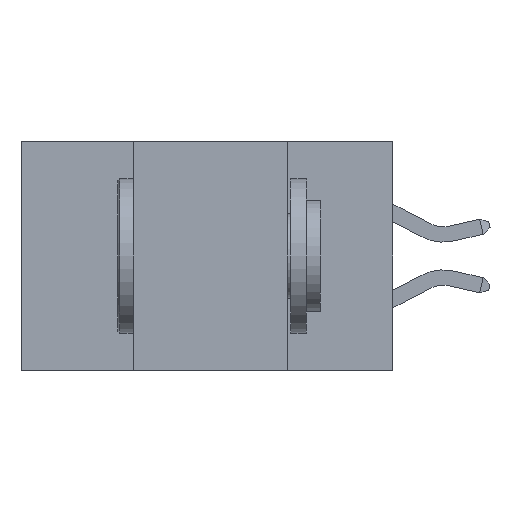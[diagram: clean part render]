
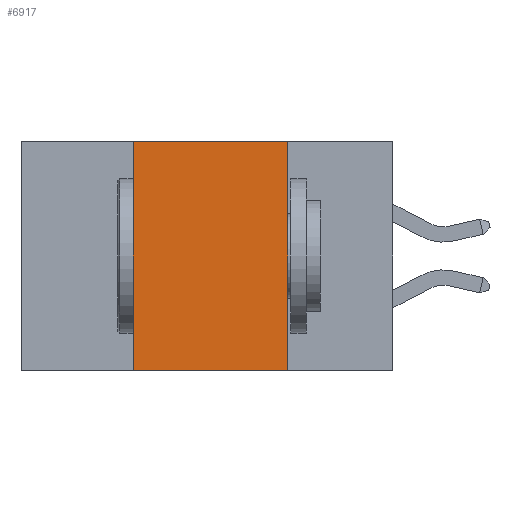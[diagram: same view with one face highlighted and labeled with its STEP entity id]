
A CAD part, left-side view. The second image highlights one B-rep face of the part: STEP entity #6917.
In plain terms, the highlighted planar face has unit normal (-1, 0, 0).
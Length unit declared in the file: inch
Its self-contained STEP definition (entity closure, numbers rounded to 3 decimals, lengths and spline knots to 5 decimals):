
#660 = VECTOR ( 'NONE', #10947, 39.37008 ) ;
#1397 = CARTESIAN_POINT ( 'NONE',  ( 0., 0.42, -0.37 ) ) ;
#1821 = VECTOR ( 'NONE', #13960, 39.37008 ) ;
#2863 = ORIENTED_EDGE ( 'NONE', *, *, #6909, .F. ) ;
#2945 = VERTEX_POINT ( 'NONE', #1397 ) ;
#3804 = FACE_OUTER_BOUND ( 'NONE', #12808, .T. ) ;
#4958 = CARTESIAN_POINT ( 'NONE',  ( 0., 0.42, 0. ) ) ;
#4995 = AXIS2_PLACEMENT_3D ( 'NONE', #10942, #10106, #10090 ) ;
#6909 = EDGE_CURVE ( 'NONE', #14402, #8915, #10139, .T. ) ;
#6917 = ADVANCED_FACE ( 'NONE', ( #3804 ), #10179, .F. ) ;
#7707 = VECTOR ( 'NONE', #7890, 39.37008 ) ;
#7890 = DIRECTION ( 'NONE',  ( 0., 0., 1. ) ) ;
#8915 = VERTEX_POINT ( 'NONE', #10567 ) ;
#8934 = ORIENTED_EDGE ( 'NONE', *, *, #9703, .F. ) ;
#9703 = EDGE_CURVE ( 'NONE', #2945, #14402, #10601, .T. ) ;
#9762 = CARTESIAN_POINT ( 'NONE',  ( 0., 0.17, 0. ) ) ;
#10090 = DIRECTION ( 'NONE',  ( 0., 0., -1. ) ) ;
#10106 = DIRECTION ( 'NONE',  ( 1., 0., 0. ) ) ;
#10139 = LINE ( 'NONE', #10422, #660 ) ;
#10179 = PLANE ( 'NONE',  #4995 ) ;
#10422 = CARTESIAN_POINT ( 'NONE',  ( 0., 0.6, 0. ) ) ;
#10567 = CARTESIAN_POINT ( 'NONE',  ( 0., 0.17, 0. ) ) ;
#10601 = LINE ( 'NONE', #12152, #7707 ) ;
#10791 = CARTESIAN_POINT ( 'NONE',  ( 0., 0.6, -0.37 ) ) ;
#10942 = CARTESIAN_POINT ( 'NONE',  ( 0., 0.6, 0. ) ) ;
#10947 = DIRECTION ( 'NONE',  ( 0., -1., 0. ) ) ;
#11433 = ORIENTED_EDGE ( 'NONE', *, *, #12025, .F. ) ;
#11765 = ORIENTED_EDGE ( 'NONE', *, *, #12648, .T. ) ;
#12025 = EDGE_CURVE ( 'NONE', #8915, #13913, #13830, .T. ) ;
#12152 = CARTESIAN_POINT ( 'NONE',  ( 0., 0.42, 0. ) ) ;
#12648 = EDGE_CURVE ( 'NONE', #2945, #13913, #13645, .T. ) ;
#12808 = EDGE_LOOP ( 'NONE', ( #11433, #2863, #8934, #11765 ) ) ;
#12944 = DIRECTION ( 'NONE',  ( 0., 0., -1. ) ) ;
#13494 = VECTOR ( 'NONE', #12944, 39.37008 ) ;
#13645 = LINE ( 'NONE', #10791, #1821 ) ;
#13701 = CARTESIAN_POINT ( 'NONE',  ( 0., 0.17, -0.37 ) ) ;
#13830 = LINE ( 'NONE', #9762, #13494 ) ;
#13913 = VERTEX_POINT ( 'NONE', #13701 ) ;
#13960 = DIRECTION ( 'NONE',  ( 0., -1., 0. ) ) ;
#14402 = VERTEX_POINT ( 'NONE', #4958 ) ;
